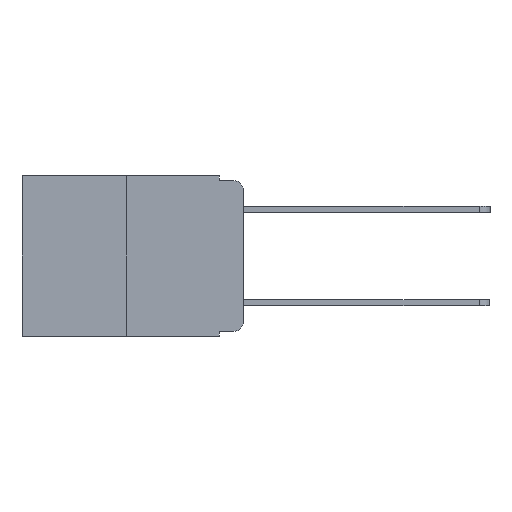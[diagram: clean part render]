
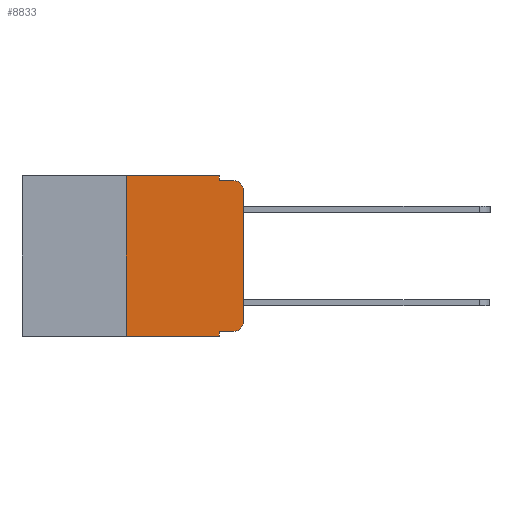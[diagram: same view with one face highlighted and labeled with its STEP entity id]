
A CAD part, left-side view. The second image highlights one B-rep face of the part: STEP entity #8833.
In plain terms, the highlighted planar face has unit normal (-1, 0, 0).
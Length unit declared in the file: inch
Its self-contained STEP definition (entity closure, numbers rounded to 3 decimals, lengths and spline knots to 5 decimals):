
#133 = CARTESIAN_POINT ( 'NONE',  ( 0., 0.02, -0.313 ) ) ;
#170 = CARTESIAN_POINT ( 'NONE',  ( 0., 0.051, -0.333 ) ) ;
#175 = VERTEX_POINT ( 'NONE', #5594 ) ;
#243 = DIRECTION ( 'NONE',  ( 0., 0., -1. ) ) ;
#694 = VERTEX_POINT ( 'NONE', #13168 ) ;
#1051 = EDGE_CURVE ( 'NONE', #12893, #13852, #3347, .T. ) ;
#1055 = VECTOR ( 'NONE', #4094, 39.37008 ) ;
#1079 = FACE_OUTER_BOUND ( 'NONE', #4215, .T. ) ;
#1225 = VECTOR ( 'NONE', #6809, 39.37008 ) ;
#1790 = EDGE_CURVE ( 'NONE', #8184, #11700, #12329, .T. ) ;
#1908 = EDGE_CURVE ( 'NONE', #14526, #13420, #4231, .T. ) ;
#2376 = ORIENTED_EDGE ( 'NONE', *, *, #12539, .T. ) ;
#2559 = EDGE_CURVE ( 'NONE', #694, #17413, #12514, .T. ) ;
#2887 = DIRECTION ( 'NONE',  ( 1., 0., 0. ) ) ;
#3243 = ORIENTED_EDGE ( 'NONE', *, *, #16656, .T. ) ;
#3347 = CIRCLE ( 'NONE', #5746, 0.02 ) ;
#3396 = CIRCLE ( 'NONE', #8267, 0.02 ) ;
#3547 = CARTESIAN_POINT ( 'NONE',  ( 0., 0.473, -0.343 ) ) ;
#4094 = DIRECTION ( 'NONE',  ( 0., -1., 0. ) ) ;
#4097 = EDGE_CURVE ( 'NONE', #175, #694, #7872, .T. ) ;
#4215 = EDGE_LOOP ( 'NONE', ( #14275, #2376, #5527, #7151, #6778, #7598, #3243, #4924, #6428, #9888 ) ) ;
#4231 = LINE ( 'NONE', #5062, #11028 ) ;
#4438 = DIRECTION ( 'NONE',  ( 0., 0., 1. ) ) ;
#4588 = EDGE_CURVE ( 'NONE', #13852, #10925, #17312, .T. ) ;
#4920 = CARTESIAN_POINT ( 'NONE',  ( 0., 0.051, -0.343 ) ) ;
#4924 = ORIENTED_EDGE ( 'NONE', *, *, #1790, .F. ) ;
#4998 = DIRECTION ( 'NONE',  ( 0., -1., 0. ) ) ;
#5062 = CARTESIAN_POINT ( 'NONE',  ( 0., 0.25, 0. ) ) ;
#5527 = ORIENTED_EDGE ( 'NONE', *, *, #2559, .F. ) ;
#5594 = CARTESIAN_POINT ( 'NONE',  ( 0., 0.051, 0. ) ) ;
#5746 = AXIS2_PLACEMENT_3D ( 'NONE', #133, #15647, #243 ) ;
#6230 = CARTESIAN_POINT ( 'NONE',  ( 0., 0.25, 0. ) ) ;
#6253 = CARTESIAN_POINT ( 'NONE',  ( 0., 0.25, -0.343 ) ) ;
#6428 = ORIENTED_EDGE ( 'NONE', *, *, #8322, .T. ) ;
#6707 = AXIS2_PLACEMENT_3D ( 'NONE', #13831, #2887, #12508 ) ;
#6778 = ORIENTED_EDGE ( 'NONE', *, *, #16836, .F. ) ;
#6809 = DIRECTION ( 'NONE',  ( 0., -1., 0. ) ) ;
#6965 = CARTESIAN_POINT ( 'NONE',  ( 0., 0.02, -0.03 ) ) ;
#7082 = LINE ( 'NONE', #170, #13413 ) ;
#7151 = ORIENTED_EDGE ( 'NONE', *, *, #4097, .F. ) ;
#7598 = ORIENTED_EDGE ( 'NONE', *, *, #1908, .F. ) ;
#7872 = LINE ( 'NONE', #14078, #14197 ) ;
#8184 = VERTEX_POINT ( 'NONE', #16374 ) ;
#8267 = AXIS2_PLACEMENT_3D ( 'NONE', #6965, #16391, #8331 ) ;
#8322 = EDGE_CURVE ( 'NONE', #8184, #12893, #7082, .T. ) ;
#8331 = DIRECTION ( 'NONE',  ( 0., 0., -1. ) ) ;
#8378 = CARTESIAN_POINT ( 'NONE',  ( 0., 0.02, -0.01 ) ) ;
#8578 = DIRECTION ( 'NONE',  ( 0., -1., 0. ) ) ;
#8732 = VECTOR ( 'NONE', #11963, 39.37008 ) ;
#8833 = ADVANCED_FACE ( 'NONE', ( #1079 ), #9749, .F. ) ;
#9748 = CARTESIAN_POINT ( 'NONE',  ( 0., 0., -0.313 ) ) ;
#9749 = PLANE ( 'NONE',  #6707 ) ;
#9888 = ORIENTED_EDGE ( 'NONE', *, *, #1051, .T. ) ;
#10925 = VERTEX_POINT ( 'NONE', #16814 ) ;
#11028 = VECTOR ( 'NONE', #13453, 39.37008 ) ;
#11389 = VECTOR ( 'NONE', #4998, 39.37008 ) ;
#11579 = CARTESIAN_POINT ( 'NONE',  ( 0., 0.051, 0. ) ) ;
#11700 = VERTEX_POINT ( 'NONE', #4920 ) ;
#11963 = DIRECTION ( 'NONE',  ( 0., 0., -1. ) ) ;
#12329 = LINE ( 'NONE', #11579, #8732 ) ;
#12508 = DIRECTION ( 'NONE',  ( 0., 0., -1. ) ) ;
#12514 = LINE ( 'NONE', #13712, #1055 ) ;
#12539 = EDGE_CURVE ( 'NONE', #10925, #17413, #3396, .T. ) ;
#12564 = CARTESIAN_POINT ( 'NONE',  ( 0., 0., 0. ) ) ;
#12695 = DIRECTION ( 'NONE',  ( 0., 0., -1. ) ) ;
#12893 = VERTEX_POINT ( 'NONE', #14507 ) ;
#13168 = CARTESIAN_POINT ( 'NONE',  ( 0., 0.051, -0.01 ) ) ;
#13413 = VECTOR ( 'NONE', #8578, 39.37008 ) ;
#13420 = VERTEX_POINT ( 'NONE', #6230 ) ;
#13453 = DIRECTION ( 'NONE',  ( 0., 0., 1. ) ) ;
#13712 = CARTESIAN_POINT ( 'NONE',  ( 0., 0.051, -0.01 ) ) ;
#13755 = VECTOR ( 'NONE', #4438, 39.37008 ) ;
#13831 = CARTESIAN_POINT ( 'NONE',  ( 0., 0.473, 0. ) ) ;
#13852 = VERTEX_POINT ( 'NONE', #9748 ) ;
#14078 = CARTESIAN_POINT ( 'NONE',  ( 0., 0.051, 0. ) ) ;
#14197 = VECTOR ( 'NONE', #12695, 39.37008 ) ;
#14275 = ORIENTED_EDGE ( 'NONE', *, *, #4588, .T. ) ;
#14507 = CARTESIAN_POINT ( 'NONE',  ( 0., 0.02, -0.333 ) ) ;
#14526 = VERTEX_POINT ( 'NONE', #6253 ) ;
#15041 = LINE ( 'NONE', #3547, #11389 ) ;
#15432 = LINE ( 'NONE', #16224, #1225 ) ;
#15647 = DIRECTION ( 'NONE',  ( -1., 0., 0. ) ) ;
#16224 = CARTESIAN_POINT ( 'NONE',  ( 0., 0.473, 0. ) ) ;
#16374 = CARTESIAN_POINT ( 'NONE',  ( 0., 0.051, -0.333 ) ) ;
#16391 = DIRECTION ( 'NONE',  ( -1., 0., 0. ) ) ;
#16656 = EDGE_CURVE ( 'NONE', #14526, #11700, #15041, .T. ) ;
#16814 = CARTESIAN_POINT ( 'NONE',  ( 0., 0., -0.03 ) ) ;
#16836 = EDGE_CURVE ( 'NONE', #13420, #175, #15432, .T. ) ;
#17312 = LINE ( 'NONE', #12564, #13755 ) ;
#17413 = VERTEX_POINT ( 'NONE', #8378 ) ;
